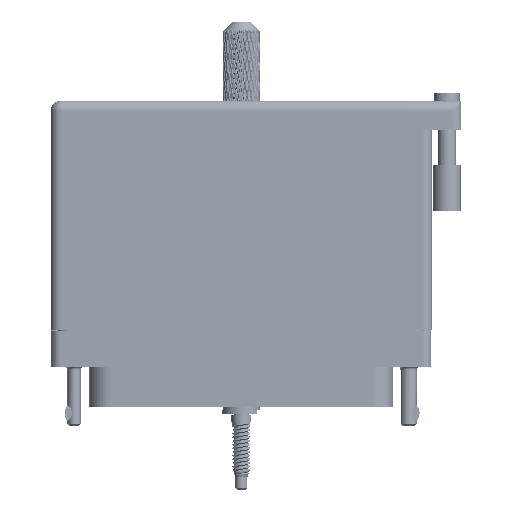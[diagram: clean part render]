
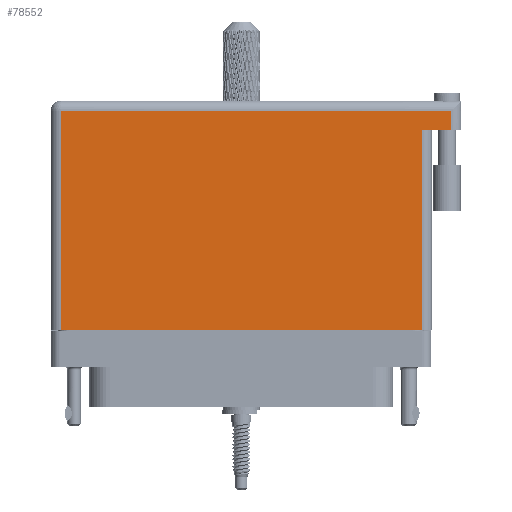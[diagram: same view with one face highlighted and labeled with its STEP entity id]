
A CAD part, front view. The second image highlights one B-rep face of the part: STEP entity #78552.
In plain terms, the highlighted face is planar.
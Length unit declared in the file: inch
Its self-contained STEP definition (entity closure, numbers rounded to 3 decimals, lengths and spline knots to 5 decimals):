
#1002 = PLANE ( 'NONE',  #105422 ) ;
#1988 = CARTESIAN_POINT ( 'NONE',  ( 1.43, 1.396, 0.4495 ) ) ;
#4308 = CARTESIAN_POINT ( 'NONE',  ( 1.5, 1.269, 0.4495 ) ) ;
#8014 = CARTESIAN_POINT ( 'NONE',  ( -1.23, -0.1, 0.4495 ) ) ;
#9736 = EDGE_CURVE ( 'NONE', #88244, #69510, #27483, .T. ) ;
#10861 = FACE_OUTER_BOUND ( 'NONE', #103888, .T. ) ;
#11473 = DIRECTION ( 'NONE',  ( 0., 1., 0. ) ) ;
#17302 = VERTEX_POINT ( 'NONE', #71383 ) ;
#17786 = DIRECTION ( 'NONE',  ( 0., -1., 0. ) ) ;
#22217 = DIRECTION ( 'NONE',  ( -1., 0., 0. ) ) ;
#23962 = CARTESIAN_POINT ( 'NONE',  ( 1.43, 1.466, 0.4495 ) ) ;
#27483 = LINE ( 'NONE', #124839, #82530 ) ;
#30878 = VECTOR ( 'NONE', #11473, 39.37008 ) ;
#42563 = EDGE_CURVE ( 'NONE', #83362, #17302, #96573, .T. ) ;
#49529 = LINE ( 'NONE', #111478, #124393 ) ;
#53667 = ORIENTED_EDGE ( 'NONE', *, *, #9736, .T. ) ;
#56279 = LINE ( 'NONE', #8014, #76196 ) ;
#57684 = EDGE_CURVE ( 'NONE', #69510, #71216, #56279, .T. ) ;
#61137 = CARTESIAN_POINT ( 'NONE',  ( -1.3, 1.466, 0.4495 ) ) ;
#61882 = CARTESIAN_POINT ( 'NONE',  ( 1.23, -0.1, 0.4495 ) ) ;
#64970 = DIRECTION ( 'NONE',  ( -1., 0., 0. ) ) ;
#66024 = VECTOR ( 'NONE', #93180, 39.37008 ) ;
#69510 = VERTEX_POINT ( 'NONE', #90329 ) ;
#69570 = ORIENTED_EDGE ( 'NONE', *, *, #114775, .T. ) ;
#70728 = ORIENTED_EDGE ( 'NONE', *, *, #42563, .T. ) ;
#71216 = VERTEX_POINT ( 'NONE', #88030 ) ;
#71383 = CARTESIAN_POINT ( 'NONE',  ( 1.23, 1.269, 0.4495 ) ) ;
#76196 = VECTOR ( 'NONE', #17786, 39.37008 ) ;
#78552 = ADVANCED_FACE ( 'NONE', ( #10861 ), #1002, .F. ) ;
#79066 = CARTESIAN_POINT ( 'NONE',  ( 1.23, 1.269, 0.4495 ) ) ;
#81539 = VECTOR ( 'NONE', #83383, 39.37008 ) ;
#82530 = VECTOR ( 'NONE', #64970, 39.37008 ) ;
#83362 = VERTEX_POINT ( 'NONE', #61882 ) ;
#83383 = DIRECTION ( 'NONE',  ( 0., 1., 0. ) ) ;
#83805 = ORIENTED_EDGE ( 'NONE', *, *, #57684, .T. ) ;
#85799 = EDGE_CURVE ( 'NONE', #104032, #88244, #107509, .T. ) ;
#88030 = CARTESIAN_POINT ( 'NONE',  ( -1.23, -0.1, 0.4495 ) ) ;
#88244 = VERTEX_POINT ( 'NONE', #1988 ) ;
#88721 = ORIENTED_EDGE ( 'NONE', *, *, #85799, .T. ) ;
#90329 = CARTESIAN_POINT ( 'NONE',  ( -1.23, 1.396, 0.4495 ) ) ;
#93180 = DIRECTION ( 'NONE',  ( -1., 0., 0. ) ) ;
#96573 = LINE ( 'NONE', #79066, #30878 ) ;
#96821 = ORIENTED_EDGE ( 'NONE', *, *, #102990, .F. ) ;
#102990 = EDGE_CURVE ( 'NONE', #104032, #17302, #111879, .T. ) ;
#103587 = CARTESIAN_POINT ( 'NONE',  ( 1.43, 1.269, 0.4495 ) ) ;
#103888 = EDGE_LOOP ( 'NONE', ( #69570, #70728, #96821, #88721, #53667, #83805 ) ) ;
#104032 = VERTEX_POINT ( 'NONE', #103587 ) ;
#105422 = AXIS2_PLACEMENT_3D ( 'NONE', #61137, #119682, #22217 ) ;
#105468 = DIRECTION ( 'NONE',  ( 1., 0., 0. ) ) ;
#107509 = LINE ( 'NONE', #23962, #81539 ) ;
#111478 = CARTESIAN_POINT ( 'NONE',  ( -1.3, -0.1, 0.4495 ) ) ;
#111879 = LINE ( 'NONE', #4308, #66024 ) ;
#114775 = EDGE_CURVE ( 'NONE', #71216, #83362, #49529, .T. ) ;
#119682 = DIRECTION ( 'NONE',  ( 0., 0., -1. ) ) ;
#124393 = VECTOR ( 'NONE', #105468, 39.37008 ) ;
#124839 = CARTESIAN_POINT ( 'NONE',  ( -1.3, 1.396, 0.4495 ) ) ;
